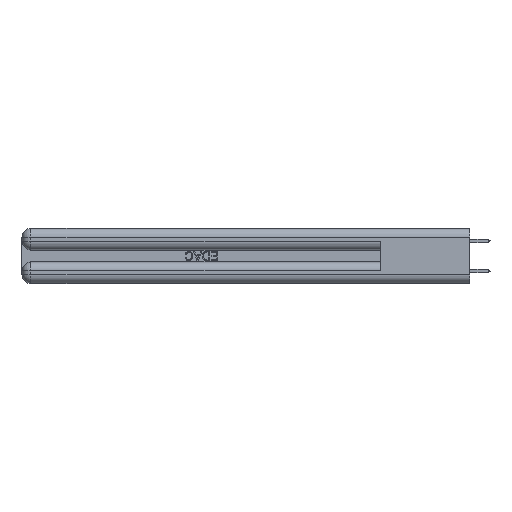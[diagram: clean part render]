
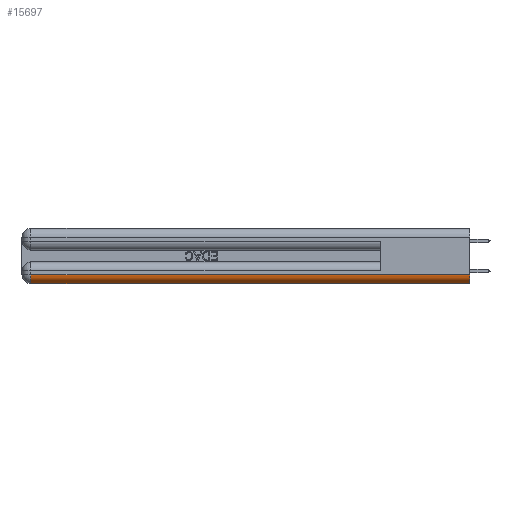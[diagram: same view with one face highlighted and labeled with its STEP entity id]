
A CAD part, left-side view. The second image highlights one B-rep face of the part: STEP entity #15697.
In plain terms, the highlighted cylindrical face has radius 1.524 mm (diameter 3.048 mm), a partial arc.
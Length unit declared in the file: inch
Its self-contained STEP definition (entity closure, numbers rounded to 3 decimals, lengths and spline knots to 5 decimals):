
#9 = CARTESIAN_POINT ( 'NONE',  ( 0.06, 3., 0. ) ) ;
#1729 = DIRECTION ( 'NONE',  ( 0., 1., 0. ) ) ;
#1769 = CARTESIAN_POINT ( 'NONE',  ( 0.06, 0., 0.06 ) ) ;
#1797 = VERTEX_POINT ( 'NONE', #16871 ) ;
#4269 = DIRECTION ( 'NONE',  ( 0., 1., 0. ) ) ;
#5685 = DIRECTION ( 'NONE',  ( 0., 0., 1. ) ) ;
#6815 = ORIENTED_EDGE ( 'NONE', *, *, #42821, .F. ) ;
#7377 = EDGE_LOOP ( 'NONE', ( #15436, #15280, #6815, #38338 ) ) ;
#7849 = CARTESIAN_POINT ( 'NONE',  ( 0.06, 0., 0.06 ) ) ;
#7936 = CIRCLE ( 'NONE', #29700, 0.06 ) ;
#8444 = VERTEX_POINT ( 'NONE', #26670 ) ;
#11509 = AXIS2_PLACEMENT_3D ( 'NONE', #7849, #4269, #27675 ) ;
#11894 = EDGE_CURVE ( 'NONE', #1797, #8444, #47723, .T. ) ;
#13267 = VECTOR ( 'NONE', #42985, 39.37008 ) ;
#15041 = FACE_OUTER_BOUND ( 'NONE', #7377, .T. ) ;
#15280 = ORIENTED_EDGE ( 'NONE', *, *, #16344, .F. ) ;
#15436 = ORIENTED_EDGE ( 'NONE', *, *, #11894, .F. ) ;
#15697 = ADVANCED_FACE ( 'NONE', ( #15041 ), #24158, .T. ) ;
#15923 = VERTEX_POINT ( 'NONE', #32963 ) ;
#16190 = CARTESIAN_POINT ( 'NONE',  ( 0., 0., 0.06 ) ) ;
#16344 = EDGE_CURVE ( 'NONE', #24213, #1797, #47880, .T. ) ;
#16871 = CARTESIAN_POINT ( 'NONE',  ( 0., 0., 0.06 ) ) ;
#18668 = AXIS2_PLACEMENT_3D ( 'NONE', #1769, #29121, #5685 ) ;
#24158 = CYLINDRICAL_SURFACE ( 'NONE', #11509, 0.06 ) ;
#24213 = VERTEX_POINT ( 'NONE', #41971 ) ;
#25136 = CARTESIAN_POINT ( 'NONE',  ( 0.06, 2.94, 0.06 ) ) ;
#26670 = CARTESIAN_POINT ( 'NONE',  ( 0.06, 0., 0. ) ) ;
#27675 = DIRECTION ( 'NONE',  ( 0., 0., 1. ) ) ;
#27785 = DIRECTION ( 'NONE',  ( 0., -1., 0. ) ) ;
#29080 = DIRECTION ( 'NONE',  ( 0., 0., 1. ) ) ;
#29121 = DIRECTION ( 'NONE',  ( 0., -1., 0. ) ) ;
#29700 = AXIS2_PLACEMENT_3D ( 'NONE', #25136, #1729, #29080 ) ;
#32963 = CARTESIAN_POINT ( 'NONE',  ( 0.06, 2.94, 0. ) ) ;
#34045 = LINE ( 'NONE', #9, #13267 ) ;
#35033 = EDGE_CURVE ( 'NONE', #8444, #15923, #34045, .T. ) ;
#38338 = ORIENTED_EDGE ( 'NONE', *, *, #35033, .F. ) ;
#41971 = CARTESIAN_POINT ( 'NONE',  ( 0., 2.94, 0.06 ) ) ;
#42821 = EDGE_CURVE ( 'NONE', #15923, #24213, #7936, .T. ) ;
#42985 = DIRECTION ( 'NONE',  ( 0., 1., 0. ) ) ;
#46663 = VECTOR ( 'NONE', #27785, 39.37008 ) ;
#47723 = CIRCLE ( 'NONE', #18668, 0.06 ) ;
#47880 = LINE ( 'NONE', #16190, #46663 ) ;
